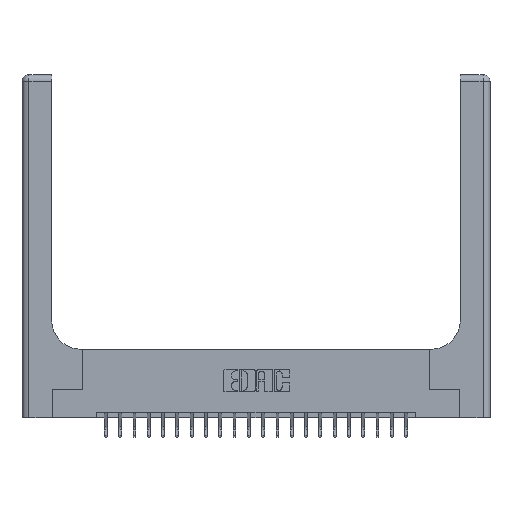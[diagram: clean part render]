
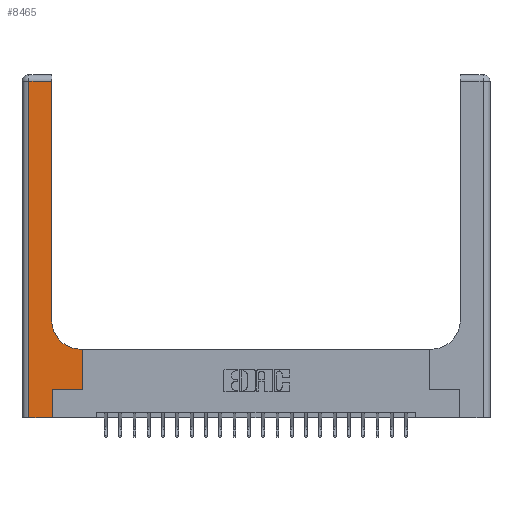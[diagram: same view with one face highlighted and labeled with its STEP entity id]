
A CAD part, top view. The second image highlights one B-rep face of the part: STEP entity #8465.
In plain terms, the highlighted planar face has unit normal (0, 0, 1).
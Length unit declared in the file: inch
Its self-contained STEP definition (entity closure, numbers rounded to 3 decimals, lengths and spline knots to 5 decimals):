
#801 = ORIENTED_EDGE ( 'NONE', *, *, #3683, .T. ) ;
#987 = DIRECTION ( 'NONE',  ( 1., 0., 0. ) ) ;
#1395 = CARTESIAN_POINT ( 'NONE',  ( 0.528, 0.6, 0.37 ) ) ;
#1526 = ORIENTED_EDGE ( 'NONE', *, *, #9165, .T. ) ;
#1706 = CARTESIAN_POINT ( 'NONE',  ( 0.51, 0.85, 0.37 ) ) ;
#1815 = CARTESIAN_POINT ( 'NONE',  ( 0.51, 0.6, 0.37 ) ) ;
#1948 = VECTOR ( 'NONE', #2405, 39.37008 ) ;
#2405 = DIRECTION ( 'NONE',  ( 0., 1., 0. ) ) ;
#2764 = VERTEX_POINT ( 'NONE', #1395 ) ;
#2774 = CARTESIAN_POINT ( 'NONE',  ( 0.265, 0., 0.37 ) ) ;
#2996 = DIRECTION ( 'NONE',  ( 0., 0., -1. ) ) ;
#3423 = ORIENTED_EDGE ( 'NONE', *, *, #5568, .T. ) ;
#3683 = EDGE_CURVE ( 'NONE', #20096, #12050, #7560, .T. ) ;
#3775 = VECTOR ( 'NONE', #18898, 39.37008 ) ;
#3808 = AXIS2_PLACEMENT_3D ( 'NONE', #1706, #2996, #15721 ) ;
#4047 = LINE ( 'NONE', #18145, #1948 ) ;
#4800 = CARTESIAN_POINT ( 'NONE',  ( 0., 2.94, 0.37 ) ) ;
#4972 = DIRECTION ( 'NONE',  ( 0., 1., 0. ) ) ;
#5213 = LINE ( 'NONE', #8683, #9010 ) ;
#5568 = EDGE_CURVE ( 'NONE', #17876, #17735, #16704, .T. ) ;
#6752 = LINE ( 'NONE', #9982, #3775 ) ;
#6881 = EDGE_CURVE ( 'NONE', #14921, #2764, #8567, .T. ) ;
#7560 = LINE ( 'NONE', #19838, #17808 ) ;
#7733 = CARTESIAN_POINT ( 'NONE',  ( 0.528, 0.25, 0.37 ) ) ;
#7906 = ORIENTED_EDGE ( 'NONE', *, *, #15150, .T. ) ;
#7958 = LINE ( 'NONE', #20108, #9784 ) ;
#8453 = CARTESIAN_POINT ( 'NONE',  ( 0.528, 0.25, 0.37 ) ) ;
#8465 = ADVANCED_FACE ( 'NONE', ( #11080 ), #19888, .F. ) ;
#8567 = LINE ( 'NONE', #8453, #16994 ) ;
#8683 = CARTESIAN_POINT ( 'NONE',  ( 0.06, 3., 0.37 ) ) ;
#9010 = VECTOR ( 'NONE', #15842, 39.37008 ) ;
#9165 = EDGE_CURVE ( 'NONE', #2764, #17876, #6752, .T. ) ;
#9206 = CARTESIAN_POINT ( 'NONE',  ( 0.06, 0., 0.37 ) ) ;
#9360 = VERTEX_POINT ( 'NONE', #22840 ) ;
#9784 = VECTOR ( 'NONE', #987, 39.37008 ) ;
#9982 = CARTESIAN_POINT ( 'NONE',  ( 0.26, 0.6, 0.37 ) ) ;
#11080 = FACE_OUTER_BOUND ( 'NONE', #17541, .T. ) ;
#12038 = DIRECTION ( 'NONE',  ( 0., 1., 0. ) ) ;
#12050 = VERTEX_POINT ( 'NONE', #19735 ) ;
#12644 = DIRECTION ( 'NONE',  ( 1., 0., 0. ) ) ;
#12793 = ORIENTED_EDGE ( 'NONE', *, *, #20876, .T. ) ;
#12974 = EDGE_CURVE ( 'NONE', #9360, #20096, #5213, .T. ) ;
#13076 = EDGE_CURVE ( 'NONE', #17735, #13657, #4047, .T. ) ;
#13657 = VERTEX_POINT ( 'NONE', #13680 ) ;
#13680 = CARTESIAN_POINT ( 'NONE',  ( 0.26, 2.94, 0.37 ) ) ;
#13692 = DIRECTION ( 'NONE',  ( -1., 0., 0. ) ) ;
#14234 = VECTOR ( 'NONE', #13692, 39.37008 ) ;
#14415 = CARTESIAN_POINT ( 'NONE',  ( 0., 3., 0.37 ) ) ;
#14633 = ORIENTED_EDGE ( 'NONE', *, *, #6881, .T. ) ;
#14921 = VERTEX_POINT ( 'NONE', #7733 ) ;
#15150 = EDGE_CURVE ( 'NONE', #20392, #14921, #7958, .T. ) ;
#15649 = EDGE_CURVE ( 'NONE', #13657, #9360, #17163, .T. ) ;
#15721 = DIRECTION ( 'NONE',  ( 1., 0., 0. ) ) ;
#15842 = DIRECTION ( 'NONE',  ( 0., -1., 0. ) ) ;
#15911 = AXIS2_PLACEMENT_3D ( 'NONE', #14415, #16042, #15923 ) ;
#15923 = DIRECTION ( 'NONE',  ( -1., 0., 0. ) ) ;
#16042 = DIRECTION ( 'NONE',  ( 0., 0., -1. ) ) ;
#16381 = VECTOR ( 'NONE', #4972, 39.37008 ) ;
#16704 = CIRCLE ( 'NONE', #3808, 0.25 ) ;
#16994 = VECTOR ( 'NONE', #12038, 39.37008 ) ;
#17163 = LINE ( 'NONE', #4800, #14234 ) ;
#17541 = EDGE_LOOP ( 'NONE', ( #22019, #19994, #19746, #801, #12793, #7906, #14633, #1526, #3423 ) ) ;
#17735 = VERTEX_POINT ( 'NONE', #20714 ) ;
#17808 = VECTOR ( 'NONE', #12644, 39.37008 ) ;
#17876 = VERTEX_POINT ( 'NONE', #1815 ) ;
#18145 = CARTESIAN_POINT ( 'NONE',  ( 0.26, 3., 0.37 ) ) ;
#18631 = LINE ( 'NONE', #2774, #16381 ) ;
#18898 = DIRECTION ( 'NONE',  ( -1., 0., 0. ) ) ;
#19735 = CARTESIAN_POINT ( 'NONE',  ( 0.265, 0., 0.37 ) ) ;
#19746 = ORIENTED_EDGE ( 'NONE', *, *, #12974, .T. ) ;
#19838 = CARTESIAN_POINT ( 'NONE',  ( 0., 0., 0.37 ) ) ;
#19888 = PLANE ( 'NONE',  #15911 ) ;
#19994 = ORIENTED_EDGE ( 'NONE', *, *, #15649, .T. ) ;
#20096 = VERTEX_POINT ( 'NONE', #9206 ) ;
#20108 = CARTESIAN_POINT ( 'NONE',  ( 0.265, 0.25, 0.37 ) ) ;
#20392 = VERTEX_POINT ( 'NONE', #20862 ) ;
#20714 = CARTESIAN_POINT ( 'NONE',  ( 0.26, 0.85, 0.37 ) ) ;
#20862 = CARTESIAN_POINT ( 'NONE',  ( 0.265, 0.25, 0.37 ) ) ;
#20876 = EDGE_CURVE ( 'NONE', #12050, #20392, #18631, .T. ) ;
#22019 = ORIENTED_EDGE ( 'NONE', *, *, #13076, .T. ) ;
#22840 = CARTESIAN_POINT ( 'NONE',  ( 0.06, 2.94, 0.37 ) ) ;
